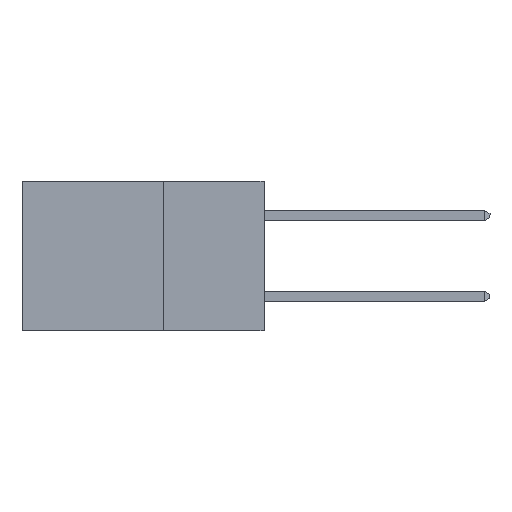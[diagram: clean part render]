
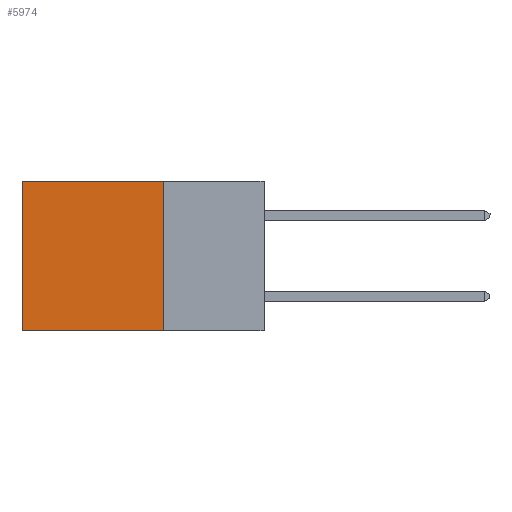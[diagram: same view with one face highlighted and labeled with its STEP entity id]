
A CAD part, left-side view. The second image highlights one B-rep face of the part: STEP entity #5974.
In plain terms, the highlighted planar face has unit normal (-1, 0, 0).
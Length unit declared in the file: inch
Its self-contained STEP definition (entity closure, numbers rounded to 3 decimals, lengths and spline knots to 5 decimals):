
#804 = LINE ( 'NONE', #3752, #12193 ) ;
#849 = LINE ( 'NONE', #10950, #6709 ) ;
#901 = PLANE ( 'NONE',  #6407 ) ;
#1687 = EDGE_CURVE ( 'NONE', #12234, #7422, #8630, .T. ) ;
#1781 = EDGE_LOOP ( 'NONE', ( #6636, #10544, #4260, #9899 ) ) ;
#2172 = LINE ( 'NONE', #4865, #4724 ) ;
#2636 = CARTESIAN_POINT ( 'NONE',  ( 0.298, 0.6, -0.37 ) ) ;
#2949 = EDGE_CURVE ( 'NONE', #12234, #4150, #2172, .T. ) ;
#3715 = DIRECTION ( 'NONE',  ( 0., 1., 0. ) ) ;
#3752 = CARTESIAN_POINT ( 'NONE',  ( 0.298, 0.6, 0. ) ) ;
#3822 = EDGE_CURVE ( 'NONE', #7422, #12942, #849, .T. ) ;
#4150 = VERTEX_POINT ( 'NONE', #12780 ) ;
#4260 = ORIENTED_EDGE ( 'NONE', *, *, #1687, .F. ) ;
#4306 = DIRECTION ( 'NONE',  ( 0., 0., -1. ) ) ;
#4724 = VECTOR ( 'NONE', #3715, 39.37008 ) ;
#4865 = CARTESIAN_POINT ( 'NONE',  ( 0.298, 0.25, 0. ) ) ;
#5604 = EDGE_CURVE ( 'NONE', #4150, #12942, #804, .T. ) ;
#5879 = DIRECTION ( 'NONE',  ( 0., 0., -1. ) ) ;
#5974 = ADVANCED_FACE ( 'NONE', ( #8345 ), #901, .F. ) ;
#6407 = AXIS2_PLACEMENT_3D ( 'NONE', #10765, #10815, #4306 ) ;
#6636 = ORIENTED_EDGE ( 'NONE', *, *, #5604, .T. ) ;
#6709 = VECTOR ( 'NONE', #11056, 39.37008 ) ;
#7422 = VERTEX_POINT ( 'NONE', #8619 ) ;
#8345 = FACE_OUTER_BOUND ( 'NONE', #1781, .T. ) ;
#8619 = CARTESIAN_POINT ( 'NONE',  ( 0.298, 0.25, -0.37 ) ) ;
#8630 = LINE ( 'NONE', #10303, #14211 ) ;
#8995 = CARTESIAN_POINT ( 'NONE',  ( 0.298, 0.25, 0. ) ) ;
#9899 = ORIENTED_EDGE ( 'NONE', *, *, #2949, .T. ) ;
#10120 = DIRECTION ( 'NONE',  ( 0., 0., -1. ) ) ;
#10303 = CARTESIAN_POINT ( 'NONE',  ( 0.298, 0.25, 0. ) ) ;
#10544 = ORIENTED_EDGE ( 'NONE', *, *, #3822, .F. ) ;
#10765 = CARTESIAN_POINT ( 'NONE',  ( 0.298, 0.25, 0. ) ) ;
#10815 = DIRECTION ( 'NONE',  ( 1., 0., 0. ) ) ;
#10950 = CARTESIAN_POINT ( 'NONE',  ( 0.298, 0.25, -0.37 ) ) ;
#11056 = DIRECTION ( 'NONE',  ( 0., 1., 0. ) ) ;
#12193 = VECTOR ( 'NONE', #5879, 39.37008 ) ;
#12234 = VERTEX_POINT ( 'NONE', #8995 ) ;
#12780 = CARTESIAN_POINT ( 'NONE',  ( 0.298, 0.6, 0. ) ) ;
#12942 = VERTEX_POINT ( 'NONE', #2636 ) ;
#14211 = VECTOR ( 'NONE', #10120, 39.37008 ) ;
